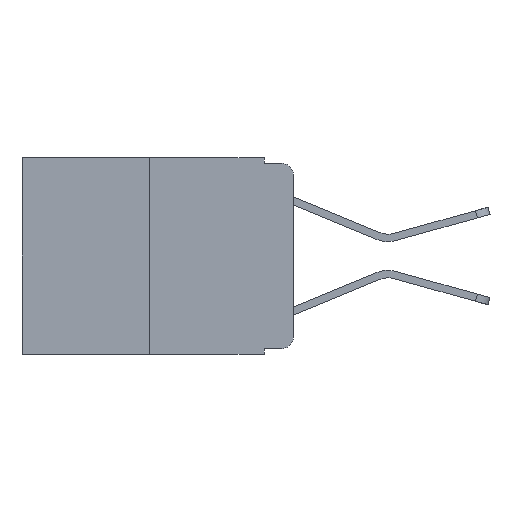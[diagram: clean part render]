
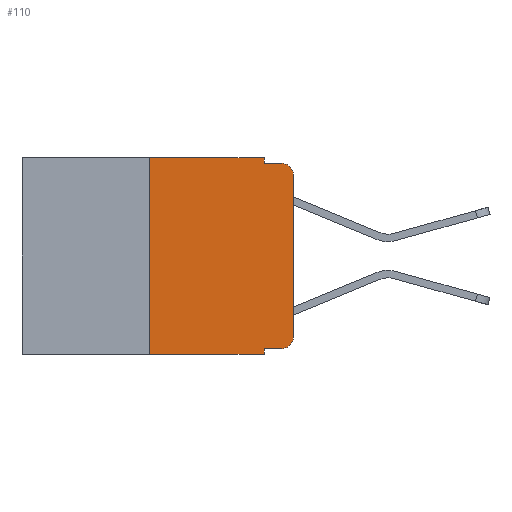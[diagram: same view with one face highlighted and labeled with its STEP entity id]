
A CAD part, left-side view. The second image highlights one B-rep face of the part: STEP entity #110.
In plain terms, the highlighted planar face has unit normal (-1, 0, 0).
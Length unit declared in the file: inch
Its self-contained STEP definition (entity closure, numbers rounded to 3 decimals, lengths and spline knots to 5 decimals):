
#26 = VERTEX_POINT ( 'NONE', #15576 ) ;
#110 = ADVANCED_FACE ( 'NONE', ( #118 ), #17581, .F. ) ;
#118 = FACE_OUTER_BOUND ( 'NONE', #12631, .T. ) ;
#526 = CARTESIAN_POINT ( 'NONE',  ( 0., 0.473, 0. ) ) ;
#784 = CARTESIAN_POINT ( 'NONE',  ( 0., 0.051, -0.333 ) ) ;
#879 = VERTEX_POINT ( 'NONE', #784 ) ;
#991 = CARTESIAN_POINT ( 'NONE',  ( 0., 0.02, -0.03 ) ) ;
#1519 = CARTESIAN_POINT ( 'NONE',  ( 0., 0.25, 0. ) ) ;
#2068 = VECTOR ( 'NONE', #2677, 39.37008 ) ;
#2523 = DIRECTION ( 'NONE',  ( 0., 0., -1. ) ) ;
#2526 = EDGE_CURVE ( 'NONE', #10851, #7268, #14180, .T. ) ;
#2570 = VERTEX_POINT ( 'NONE', #9674 ) ;
#2677 = DIRECTION ( 'NONE',  ( 0., 0., -1. ) ) ;
#2708 = CARTESIAN_POINT ( 'NONE',  ( 0., 0.051, 0. ) ) ;
#2754 = LINE ( 'NONE', #3906, #11633 ) ;
#2946 = EDGE_CURVE ( 'NONE', #11819, #10851, #11202, .T. ) ;
#3634 = DIRECTION ( 'NONE',  ( -1., 0., 0. ) ) ;
#3687 = DIRECTION ( 'NONE',  ( 0., 0., 1. ) ) ;
#3789 = EDGE_CURVE ( 'NONE', #11819, #14058, #10445, .T. ) ;
#3906 = CARTESIAN_POINT ( 'NONE',  ( 0., 0., 0. ) ) ;
#4345 = ORIENTED_EDGE ( 'NONE', *, *, #2946, .F. ) ;
#5328 = VECTOR ( 'NONE', #17416, 39.37008 ) ;
#5403 = DIRECTION ( 'NONE',  ( 0., 0., -1. ) ) ;
#5599 = EDGE_CURVE ( 'NONE', #12179, #6251, #18776, .T. ) ;
#5820 = CARTESIAN_POINT ( 'NONE',  ( 0., 0.473, -0.343 ) ) ;
#5947 = CARTESIAN_POINT ( 'NONE',  ( 0., 0.051, -0.01 ) ) ;
#6251 = VERTEX_POINT ( 'NONE', #18839 ) ;
#6337 = VECTOR ( 'NONE', #13072, 39.37008 ) ;
#6983 = CIRCLE ( 'NONE', #18143, 0.02 ) ;
#7146 = AXIS2_PLACEMENT_3D ( 'NONE', #991, #11460, #2523 ) ;
#7222 = CARTESIAN_POINT ( 'NONE',  ( 0., 0.051, -0.333 ) ) ;
#7262 = VECTOR ( 'NONE', #3687, 39.37008 ) ;
#7268 = VERTEX_POINT ( 'NONE', #16488 ) ;
#7536 = LINE ( 'NONE', #5947, #8011 ) ;
#8011 = VECTOR ( 'NONE', #16223, 39.37008 ) ;
#8037 = ORIENTED_EDGE ( 'NONE', *, *, #9984, .F. ) ;
#8184 = ORIENTED_EDGE ( 'NONE', *, *, #2526, .F. ) ;
#8356 = EDGE_CURVE ( 'NONE', #879, #14058, #13484, .T. ) ;
#8668 = VECTOR ( 'NONE', #16000, 39.37008 ) ;
#9343 = ORIENTED_EDGE ( 'NONE', *, *, #5599, .T. ) ;
#9394 = ORIENTED_EDGE ( 'NONE', *, *, #3789, .T. ) ;
#9437 = CARTESIAN_POINT ( 'NONE',  ( 0., 0.473, 0. ) ) ;
#9601 = CARTESIAN_POINT ( 'NONE',  ( 0., 0., -0.03 ) ) ;
#9644 = DIRECTION ( 'NONE',  ( 1., 0., 0. ) ) ;
#9674 = CARTESIAN_POINT ( 'NONE',  ( 0., 0., -0.313 ) ) ;
#9984 = EDGE_CURVE ( 'NONE', #7268, #26, #13184, .T. ) ;
#10445 = LINE ( 'NONE', #5820, #17684 ) ;
#10634 = CARTESIAN_POINT ( 'NONE',  ( 0., 0.02, -0.333 ) ) ;
#10851 = VERTEX_POINT ( 'NONE', #16521 ) ;
#11202 = LINE ( 'NONE', #1519, #7262 ) ;
#11460 = DIRECTION ( 'NONE',  ( -1., 0., 0. ) ) ;
#11619 = CARTESIAN_POINT ( 'NONE',  ( 0., 0.051, 0. ) ) ;
#11633 = VECTOR ( 'NONE', #12818, 39.37008 ) ;
#11819 = VERTEX_POINT ( 'NONE', #15851 ) ;
#12077 = VERTEX_POINT ( 'NONE', #10634 ) ;
#12179 = VERTEX_POINT ( 'NONE', #9601 ) ;
#12462 = ORIENTED_EDGE ( 'NONE', *, *, #8356, .F. ) ;
#12544 = CARTESIAN_POINT ( 'NONE',  ( 0., 0.02, -0.313 ) ) ;
#12631 = EDGE_LOOP ( 'NONE', ( #12895, #9343, #17666, #8037, #8184, #4345, #9394, #12462, #14298, #18572 ) ) ;
#12818 = DIRECTION ( 'NONE',  ( 0., 0., 1. ) ) ;
#12895 = ORIENTED_EDGE ( 'NONE', *, *, #14494, .T. ) ;
#12908 = EDGE_CURVE ( 'NONE', #26, #6251, #7536, .T. ) ;
#13072 = DIRECTION ( 'NONE',  ( 0., -1., 0. ) ) ;
#13184 = LINE ( 'NONE', #2708, #5328 ) ;
#13271 = CARTESIAN_POINT ( 'NONE',  ( 0., 0.051, -0.343 ) ) ;
#13484 = LINE ( 'NONE', #11619, #2068 ) ;
#13491 = AXIS2_PLACEMENT_3D ( 'NONE', #526, #9644, #5403 ) ;
#13994 = EDGE_CURVE ( 'NONE', #879, #12077, #16429, .T. ) ;
#14003 = DIRECTION ( 'NONE',  ( 0., 0., -1. ) ) ;
#14058 = VERTEX_POINT ( 'NONE', #13271 ) ;
#14180 = LINE ( 'NONE', #9437, #6337 ) ;
#14298 = ORIENTED_EDGE ( 'NONE', *, *, #13994, .T. ) ;
#14494 = EDGE_CURVE ( 'NONE', #2570, #12179, #2754, .T. ) ;
#14650 = DIRECTION ( 'NONE',  ( 0., -1., 0. ) ) ;
#15576 = CARTESIAN_POINT ( 'NONE',  ( 0., 0.051, -0.01 ) ) ;
#15808 = EDGE_CURVE ( 'NONE', #12077, #2570, #6983, .T. ) ;
#15851 = CARTESIAN_POINT ( 'NONE',  ( 0., 0.25, -0.343 ) ) ;
#16000 = DIRECTION ( 'NONE',  ( 0., -1., 0. ) ) ;
#16223 = DIRECTION ( 'NONE',  ( 0., -1., 0. ) ) ;
#16429 = LINE ( 'NONE', #7222, #8668 ) ;
#16488 = CARTESIAN_POINT ( 'NONE',  ( 0., 0.051, 0. ) ) ;
#16521 = CARTESIAN_POINT ( 'NONE',  ( 0., 0.25, 0. ) ) ;
#17416 = DIRECTION ( 'NONE',  ( 0., 0., -1. ) ) ;
#17581 = PLANE ( 'NONE',  #13491 ) ;
#17666 = ORIENTED_EDGE ( 'NONE', *, *, #12908, .F. ) ;
#17684 = VECTOR ( 'NONE', #14650, 39.37008 ) ;
#18143 = AXIS2_PLACEMENT_3D ( 'NONE', #12544, #3634, #14003 ) ;
#18572 = ORIENTED_EDGE ( 'NONE', *, *, #15808, .T. ) ;
#18776 = CIRCLE ( 'NONE', #7146, 0.02 ) ;
#18839 = CARTESIAN_POINT ( 'NONE',  ( 0., 0.02, -0.01 ) ) ;
